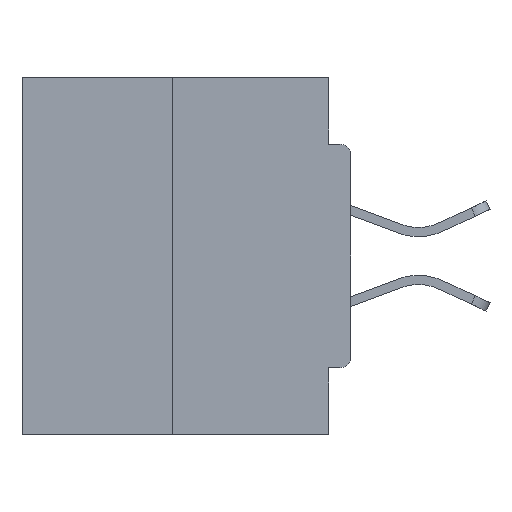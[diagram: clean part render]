
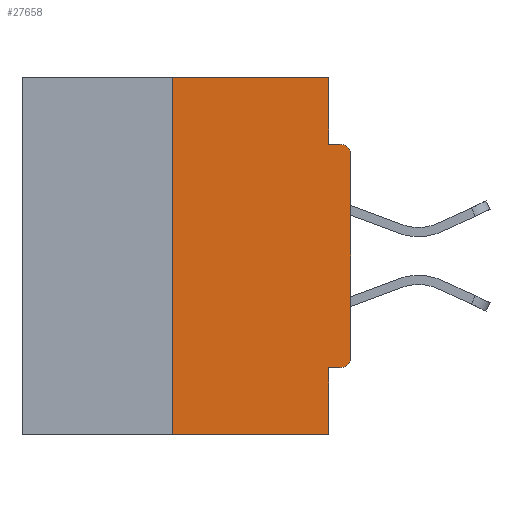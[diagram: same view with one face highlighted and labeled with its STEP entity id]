
A CAD part, left-side view. The second image highlights one B-rep face of the part: STEP entity #27658.
In plain terms, the highlighted planar face has unit normal (-1, 0, 0).
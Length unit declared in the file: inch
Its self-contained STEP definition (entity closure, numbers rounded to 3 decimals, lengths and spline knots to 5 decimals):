
#871 = EDGE_CURVE ( 'NONE', #30650, #13187, #1899, .T. ) ;
#927 = DIRECTION ( 'NONE',  ( 0., 0., -1. ) ) ;
#1479 = CARTESIAN_POINT ( 'NONE',  ( 0., 0.25, 0. ) ) ;
#1899 = LINE ( 'NONE', #26310, #14521 ) ;
#3029 = EDGE_CURVE ( 'NONE', #11180, #31922, #17602, .T. ) ;
#3110 = EDGE_CURVE ( 'NONE', #24729, #30650, #6563, .T. ) ;
#3421 = CARTESIAN_POINT ( 'NONE',  ( 0., 0.031, 0. ) ) ;
#3423 = CARTESIAN_POINT ( 'NONE',  ( 0., 0.015, -0.4065 ) ) ;
#3939 = CARTESIAN_POINT ( 'NONE',  ( 0., 0.031, -0.4065 ) ) ;
#4228 = ORIENTED_EDGE ( 'NONE', *, *, #5476, .F. ) ;
#4317 = ORIENTED_EDGE ( 'NONE', *, *, #3110, .F. ) ;
#4583 = VECTOR ( 'NONE', #927, 39.37008 ) ;
#4622 = CARTESIAN_POINT ( 'NONE',  ( 0., 0.46, 0. ) ) ;
#4843 = VECTOR ( 'NONE', #21409, 39.37008 ) ;
#5476 = EDGE_CURVE ( 'NONE', #31891, #28039, #28499, .T. ) ;
#5653 = PLANE ( 'NONE',  #23478 ) ;
#6563 = LINE ( 'NONE', #1479, #32576 ) ;
#6572 = CARTESIAN_POINT ( 'NONE',  ( 0., 0.015, -0.3915 ) ) ;
#6689 = CARTESIAN_POINT ( 'NONE',  ( 0., 0.25, 0. ) ) ;
#7200 = CIRCLE ( 'NONE', #19538, 0.015 ) ;
#8498 = CARTESIAN_POINT ( 'NONE',  ( 0., 0., -0.0935 ) ) ;
#8741 = CARTESIAN_POINT ( 'NONE',  ( 0., 0.031, -0.5 ) ) ;
#9234 = CARTESIAN_POINT ( 'NONE',  ( 0., 0.25, -0.5 ) ) ;
#10902 = VERTEX_POINT ( 'NONE', #3939 ) ;
#11154 = ORIENTED_EDGE ( 'NONE', *, *, #25062, .T. ) ;
#11180 = VERTEX_POINT ( 'NONE', #14897 ) ;
#11429 = EDGE_CURVE ( 'NONE', #10902, #25828, #19481, .T. ) ;
#11467 = VERTEX_POINT ( 'NONE', #3423 ) ;
#12370 = LINE ( 'NONE', #24097, #28983 ) ;
#12564 = DIRECTION ( 'NONE',  ( -1., 0., 0. ) ) ;
#12593 = AXIS2_PLACEMENT_3D ( 'NONE', #6572, #14178, #31824 ) ;
#12657 = ORIENTED_EDGE ( 'NONE', *, *, #22718, .F. ) ;
#13080 = DIRECTION ( 'NONE',  ( 0., 0., 1. ) ) ;
#13187 = VERTEX_POINT ( 'NONE', #31728 ) ;
#13495 = VECTOR ( 'NONE', #18410, 39.37008 ) ;
#13558 = DIRECTION ( 'NONE',  ( 0., -1., 0. ) ) ;
#13720 = DIRECTION ( 'NONE',  ( 1., 0., 0. ) ) ;
#14178 = DIRECTION ( 'NONE',  ( -1., 0., 0. ) ) ;
#14521 = VECTOR ( 'NONE', #13558, 39.37008 ) ;
#14782 = ORIENTED_EDGE ( 'NONE', *, *, #3029, .T. ) ;
#14897 = CARTESIAN_POINT ( 'NONE',  ( 0., 0., -0.3915 ) ) ;
#15095 = CARTESIAN_POINT ( 'NONE',  ( 0., 0.015, -0.1085 ) ) ;
#15621 = EDGE_CURVE ( 'NONE', #11467, #10902, #12370, .T. ) ;
#16269 = CIRCLE ( 'NONE', #12593, 0.015 ) ;
#16311 = CARTESIAN_POINT ( 'NONE',  ( 0., 0., -0.1085 ) ) ;
#16653 = VECTOR ( 'NONE', #25054, 39.37008 ) ;
#17473 = ORIENTED_EDGE ( 'NONE', *, *, #871, .F. ) ;
#17566 = CARTESIAN_POINT ( 'NONE',  ( 0., 0.46, -0.5 ) ) ;
#17602 = LINE ( 'NONE', #23196, #25893 ) ;
#18410 = DIRECTION ( 'NONE',  ( 0., -1., 0. ) ) ;
#18943 = ORIENTED_EDGE ( 'NONE', *, *, #11429, .F. ) ;
#19481 = LINE ( 'NONE', #8741, #4843 ) ;
#19538 = AXIS2_PLACEMENT_3D ( 'NONE', #15095, #12564, #22480 ) ;
#20437 = ORIENTED_EDGE ( 'NONE', *, *, #29619, .T. ) ;
#21162 = CARTESIAN_POINT ( 'NONE',  ( 0., 0.031, -0.0935 ) ) ;
#21409 = DIRECTION ( 'NONE',  ( 0., 0., -1. ) ) ;
#22480 = DIRECTION ( 'NONE',  ( 0., 0., -1. ) ) ;
#22718 = EDGE_CURVE ( 'NONE', #13187, #31891, #26288, .T. ) ;
#23065 = FACE_OUTER_BOUND ( 'NONE', #24466, .T. ) ;
#23196 = CARTESIAN_POINT ( 'NONE',  ( 0., 0., 0. ) ) ;
#23478 = AXIS2_PLACEMENT_3D ( 'NONE', #4622, #13720, #26253 ) ;
#24097 = CARTESIAN_POINT ( 'NONE',  ( 0., 0., -0.4065 ) ) ;
#24258 = DIRECTION ( 'NONE',  ( 0., 0., 1. ) ) ;
#24432 = CARTESIAN_POINT ( 'NONE',  ( 0., 0.015, -0.0935 ) ) ;
#24466 = EDGE_LOOP ( 'NONE', ( #17473, #4317, #11154, #18943, #32374, #31187, #14782, #20437, #4228, #12657 ) ) ;
#24672 = EDGE_CURVE ( 'NONE', #11467, #11180, #16269, .T. ) ;
#24729 = VERTEX_POINT ( 'NONE', #9234 ) ;
#25054 = DIRECTION ( 'NONE',  ( 0., -1., 0. ) ) ;
#25062 = EDGE_CURVE ( 'NONE', #24729, #25828, #27702, .T. ) ;
#25828 = VERTEX_POINT ( 'NONE', #31211 ) ;
#25893 = VECTOR ( 'NONE', #13080, 39.37008 ) ;
#26253 = DIRECTION ( 'NONE',  ( 0., 0., -1. ) ) ;
#26288 = LINE ( 'NONE', #3421, #4583 ) ;
#26310 = CARTESIAN_POINT ( 'NONE',  ( 0., 0.46, 0. ) ) ;
#27658 = ADVANCED_FACE ( 'NONE', ( #23065 ), #5653, .F. ) ;
#27702 = LINE ( 'NONE', #17566, #16653 ) ;
#28039 = VERTEX_POINT ( 'NONE', #24432 ) ;
#28499 = LINE ( 'NONE', #8498, #13495 ) ;
#28983 = VECTOR ( 'NONE', #32048, 39.37008 ) ;
#29619 = EDGE_CURVE ( 'NONE', #31922, #28039, #7200, .T. ) ;
#30650 = VERTEX_POINT ( 'NONE', #6689 ) ;
#31187 = ORIENTED_EDGE ( 'NONE', *, *, #24672, .T. ) ;
#31211 = CARTESIAN_POINT ( 'NONE',  ( 0., 0.031, -0.5 ) ) ;
#31728 = CARTESIAN_POINT ( 'NONE',  ( 0., 0.031, 0. ) ) ;
#31824 = DIRECTION ( 'NONE',  ( 0., 0., -1. ) ) ;
#31891 = VERTEX_POINT ( 'NONE', #21162 ) ;
#31922 = VERTEX_POINT ( 'NONE', #16311 ) ;
#32048 = DIRECTION ( 'NONE',  ( 0., 1., 0. ) ) ;
#32374 = ORIENTED_EDGE ( 'NONE', *, *, #15621, .F. ) ;
#32576 = VECTOR ( 'NONE', #24258, 39.37008 ) ;
